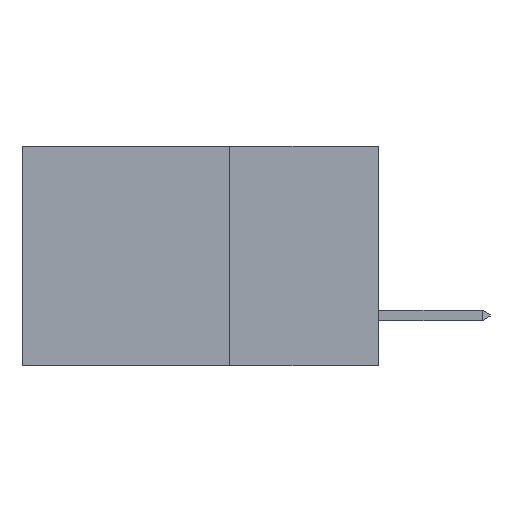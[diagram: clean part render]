
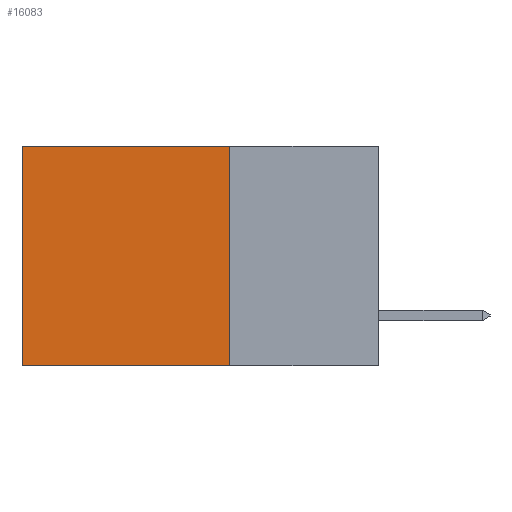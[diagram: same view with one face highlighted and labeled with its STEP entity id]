
A CAD part, left-side view. The second image highlights one B-rep face of the part: STEP entity #16083.
In plain terms, the highlighted planar face has unit normal (-1, 0, 0).
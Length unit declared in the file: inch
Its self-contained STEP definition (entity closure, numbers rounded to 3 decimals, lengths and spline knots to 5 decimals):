
#220 = CARTESIAN_POINT ( 'NONE',  ( 0.2615, 0.6, -0.37 ) ) ;
#603 = VECTOR ( 'NONE', #6627, 39.37008 ) ;
#1428 = EDGE_CURVE ( 'NONE', #7014, #3866, #8817, .T. ) ;
#1987 = ORIENTED_EDGE ( 'NONE', *, *, #8518, .F. ) ;
#2421 = DIRECTION ( 'NONE',  ( 1., 0., 0. ) ) ;
#2498 = VECTOR ( 'NONE', #12209, 39.37008 ) ;
#3866 = VERTEX_POINT ( 'NONE', #17409 ) ;
#4555 = ORIENTED_EDGE ( 'NONE', *, *, #8941, .T. ) ;
#4589 = CARTESIAN_POINT ( 'NONE',  ( 0.2615, 0.25, -0.37 ) ) ;
#5004 = LINE ( 'NONE', #4589, #12766 ) ;
#5470 = AXIS2_PLACEMENT_3D ( 'NONE', #17613, #2421, #13221 ) ;
#5682 = EDGE_CURVE ( 'NONE', #5819, #3866, #10790, .T. ) ;
#5801 = EDGE_LOOP ( 'NONE', ( #17692, #14566, #1987, #4555 ) ) ;
#5819 = VERTEX_POINT ( 'NONE', #9927 ) ;
#6627 = DIRECTION ( 'NONE',  ( 0., 0., -1. ) ) ;
#7014 = VERTEX_POINT ( 'NONE', #13783 ) ;
#7675 = CARTESIAN_POINT ( 'NONE',  ( 0.2615, 0.25, 0. ) ) ;
#7775 = FACE_OUTER_BOUND ( 'NONE', #5801, .T. ) ;
#8213 = VERTEX_POINT ( 'NONE', #7675 ) ;
#8518 = EDGE_CURVE ( 'NONE', #8213, #5819, #5004, .T. ) ;
#8817 = LINE ( 'NONE', #220, #603 ) ;
#8941 = EDGE_CURVE ( 'NONE', #8213, #7014, #13695, .T. ) ;
#9927 = CARTESIAN_POINT ( 'NONE',  ( 0.2615, 0.25, -0.37 ) ) ;
#10790 = LINE ( 'NONE', #12275, #2498 ) ;
#12209 = DIRECTION ( 'NONE',  ( 0., 1., 0. ) ) ;
#12275 = CARTESIAN_POINT ( 'NONE',  ( 0.2615, 0.25, -0.37 ) ) ;
#12766 = VECTOR ( 'NONE', #17017, 39.37008 ) ;
#13217 = VECTOR ( 'NONE', #13338, 39.37008 ) ;
#13221 = DIRECTION ( 'NONE',  ( 0., 0., -1. ) ) ;
#13338 = DIRECTION ( 'NONE',  ( 0., 1., 0. ) ) ;
#13450 = CARTESIAN_POINT ( 'NONE',  ( 0.2615, 0.25, 0. ) ) ;
#13695 = LINE ( 'NONE', #13450, #13217 ) ;
#13783 = CARTESIAN_POINT ( 'NONE',  ( 0.2615, 0.6, 0. ) ) ;
#14566 = ORIENTED_EDGE ( 'NONE', *, *, #5682, .F. ) ;
#14680 = PLANE ( 'NONE',  #5470 ) ;
#16083 = ADVANCED_FACE ( 'NONE', ( #7775 ), #14680, .F. ) ;
#17017 = DIRECTION ( 'NONE',  ( 0., 0., -1. ) ) ;
#17409 = CARTESIAN_POINT ( 'NONE',  ( 0.2615, 0.6, -0.37 ) ) ;
#17613 = CARTESIAN_POINT ( 'NONE',  ( 0.2615, 0.25, -0.37 ) ) ;
#17692 = ORIENTED_EDGE ( 'NONE', *, *, #1428, .T. ) ;
